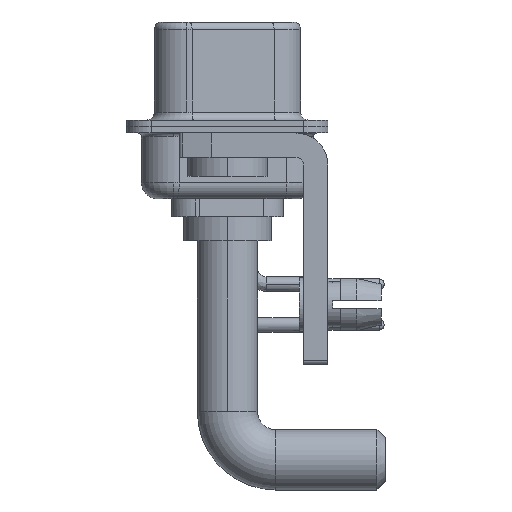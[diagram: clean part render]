
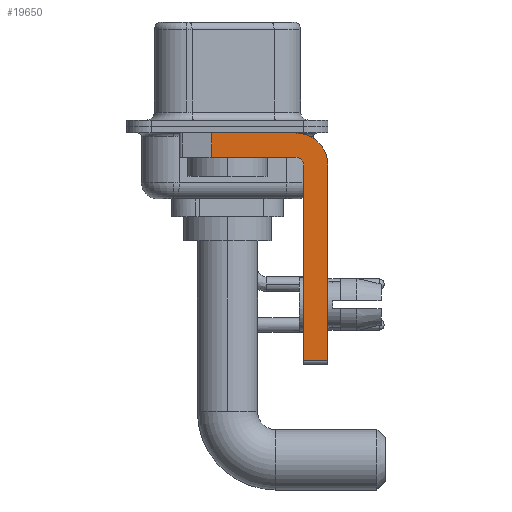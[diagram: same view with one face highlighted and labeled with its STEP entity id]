
A CAD part, left-side view. The second image highlights one B-rep face of the part: STEP entity #19650.
In plain terms, the highlighted planar face has unit normal (-1, 0, 0).
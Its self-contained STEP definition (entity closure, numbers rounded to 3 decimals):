
#30 = CIRCLE ( 'NONE', #23165, 2. ) ;
#93 = ORIENTED_EDGE ( 'NONE', *, *, #19000, .T. ) ;
#158 = VERTEX_POINT ( 'NONE', #27667 ) ;
#175 = ORIENTED_EDGE ( 'NONE', *, *, #17595, .F. ) ;
#912 = CARTESIAN_POINT ( 'NONE',  ( -2.9, -4.25, -2.4 ) ) ;
#1109 = CARTESIAN_POINT ( 'NONE',  ( -2.9, -6.25, -2.4 ) ) ;
#1339 = DIRECTION ( 'NONE',  ( 0., 1., 0. ) ) ;
#2038 = VERTEX_POINT ( 'NONE', #17912 ) ;
#3127 = FACE_OUTER_BOUND ( 'NONE', #7683, .T. ) ;
#3719 = DIRECTION ( 'NONE',  ( 0., 0., -1. ) ) ;
#3835 = DIRECTION ( 'NONE',  ( 0., 0., 1. ) ) ;
#4451 = LINE ( 'NONE', #11859, #15200 ) ;
#4471 = LINE ( 'NONE', #6487, #22018 ) ;
#4743 = VERTEX_POINT ( 'NONE', #23528 ) ;
#5749 = CARTESIAN_POINT ( 'NONE',  ( -2.9, 0.978, -0.4 ) ) ;
#6487 = CARTESIAN_POINT ( 'NONE',  ( -2.9, 3., -0.4 ) ) ;
#6838 = EDGE_CURVE ( 'NONE', #22185, #2038, #25917, .T. ) ;
#7683 = EDGE_LOOP ( 'NONE', ( #28544, #93, #23703, #175, #27424, #21193, #21815, #23922 ) ) ;
#7965 = CARTESIAN_POINT ( 'NONE',  ( -2.9, -4.25, -1.9 ) ) ;
#8639 = EDGE_CURVE ( 'NONE', #158, #4743, #30, .T. ) ;
#8813 = AXIS2_PLACEMENT_3D ( 'NONE', #10235, #12704, #22103 ) ;
#8834 = VECTOR ( 'NONE', #18528, 1000. ) ;
#10235 = CARTESIAN_POINT ( 'NONE',  ( -2.9, -4.25, -2.4 ) ) ;
#11548 = DIRECTION ( 'NONE',  ( 0., 0., -1. ) ) ;
#11859 = CARTESIAN_POINT ( 'NONE',  ( -2.9, 0.978, -1.9 ) ) ;
#12704 = DIRECTION ( 'NONE',  ( 1., 0., 0. ) ) ;
#13076 = LINE ( 'NONE', #22470, #20501 ) ;
#13314 = EDGE_CURVE ( 'NONE', #26930, #19386, #13076, .T. ) ;
#14298 = EDGE_CURVE ( 'NONE', #19517, #158, #4471, .T. ) ;
#14918 = CARTESIAN_POINT ( 'NONE',  ( -2.9, -4.75, -14.55 ) ) ;
#15200 = VECTOR ( 'NONE', #11548, 1000. ) ;
#15202 = CIRCLE ( 'NONE', #17670, 0.5 ) ;
#15899 = DIRECTION ( 'NONE',  ( 0., -1., 0. ) ) ;
#17339 = PLANE ( 'NONE',  #8813 ) ;
#17595 = EDGE_CURVE ( 'NONE', #20120, #26930, #15202, .T. ) ;
#17670 = AXIS2_PLACEMENT_3D ( 'NONE', #912, #22338, #3835 ) ;
#17912 = CARTESIAN_POINT ( 'NONE',  ( -2.9, -6.25, -14.55 ) ) ;
#18528 = DIRECTION ( 'NONE',  ( 0., -1., 0. ) ) ;
#19000 = EDGE_CURVE ( 'NONE', #19517, #19386, #4451, .T. ) ;
#19386 = VERTEX_POINT ( 'NONE', #23366 ) ;
#19517 = VERTEX_POINT ( 'NONE', #5749 ) ;
#19650 = ADVANCED_FACE ( 'NONE', ( #3127 ), #17339, .F. ) ;
#20120 = VERTEX_POINT ( 'NONE', #20205 ) ;
#20205 = CARTESIAN_POINT ( 'NONE',  ( -2.9, -4.75, -2.4 ) ) ;
#20313 = CARTESIAN_POINT ( 'NONE',  ( -2.9, -4.75, -14.8 ) ) ;
#20501 = VECTOR ( 'NONE', #1339, 1000. ) ;
#21118 = VECTOR ( 'NONE', #24482, 1000. ) ;
#21193 = ORIENTED_EDGE ( 'NONE', *, *, #6838, .T. ) ;
#21433 = CARTESIAN_POINT ( 'NONE',  ( -2.9, -4.25, -14.55 ) ) ;
#21815 = ORIENTED_EDGE ( 'NONE', *, *, #26219, .F. ) ;
#22018 = VECTOR ( 'NONE', #15899, 1000. ) ;
#22103 = DIRECTION ( 'NONE',  ( 0., 0., -1. ) ) ;
#22185 = VERTEX_POINT ( 'NONE', #14918 ) ;
#22338 = DIRECTION ( 'NONE',  ( -1., 0., 0. ) ) ;
#22470 = CARTESIAN_POINT ( 'NONE',  ( -2.9, -4.25, -1.9 ) ) ;
#23165 = AXIS2_PLACEMENT_3D ( 'NONE', #26075, #28373, #23599 ) ;
#23366 = CARTESIAN_POINT ( 'NONE',  ( -2.9, 0.978, -1.9 ) ) ;
#23528 = CARTESIAN_POINT ( 'NONE',  ( -2.9, -6.25, -2.4 ) ) ;
#23599 = DIRECTION ( 'NONE',  ( 0., 0., -1. ) ) ;
#23703 = ORIENTED_EDGE ( 'NONE', *, *, #13314, .F. ) ;
#23922 = ORIENTED_EDGE ( 'NONE', *, *, #8639, .F. ) ;
#24482 = DIRECTION ( 'NONE',  ( 0., 0., 1. ) ) ;
#24857 = LINE ( 'NONE', #1109, #25348 ) ;
#25348 = VECTOR ( 'NONE', #3719, 1000. ) ;
#25917 = LINE ( 'NONE', #21433, #8834 ) ;
#26075 = CARTESIAN_POINT ( 'NONE',  ( -2.9, -4.25, -2.4 ) ) ;
#26219 = EDGE_CURVE ( 'NONE', #4743, #2038, #24857, .T. ) ;
#26930 = VERTEX_POINT ( 'NONE', #7965 ) ;
#27424 = ORIENTED_EDGE ( 'NONE', *, *, #30120, .F. ) ;
#27667 = CARTESIAN_POINT ( 'NONE',  ( -2.9, -4.25, -0.4 ) ) ;
#28373 = DIRECTION ( 'NONE',  ( 1., 0., 0. ) ) ;
#28544 = ORIENTED_EDGE ( 'NONE', *, *, #14298, .F. ) ;
#29722 = LINE ( 'NONE', #20313, #21118 ) ;
#30120 = EDGE_CURVE ( 'NONE', #22185, #20120, #29722, .T. ) ;
